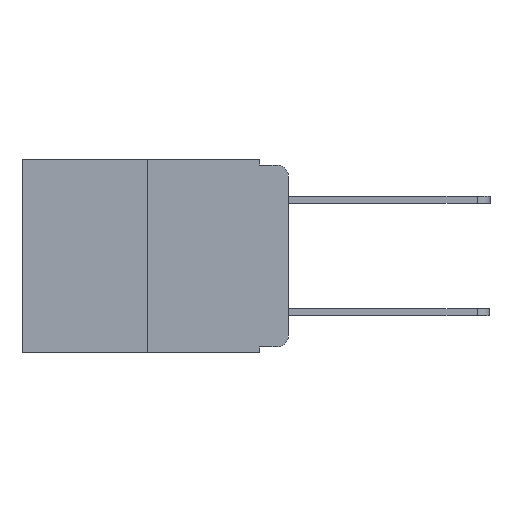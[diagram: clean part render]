
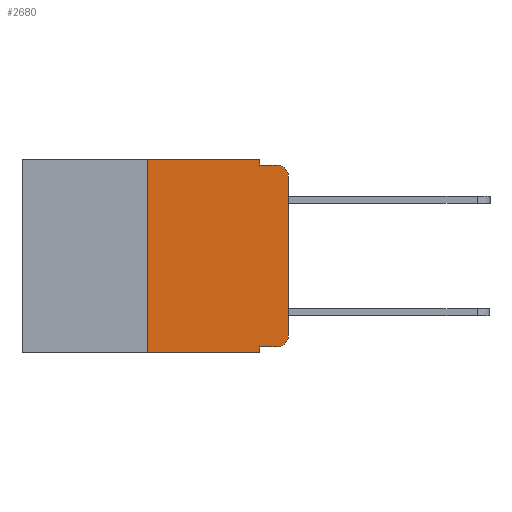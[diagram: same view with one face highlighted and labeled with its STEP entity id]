
A CAD part, left-side view. The second image highlights one B-rep face of the part: STEP entity #2680.
In plain terms, the highlighted planar face has unit normal (-1, 0, 0).
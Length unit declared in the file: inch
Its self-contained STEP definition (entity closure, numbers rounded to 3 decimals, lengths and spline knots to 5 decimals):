
#266 = DIRECTION ( 'NONE',  ( 1., 0., 0. ) ) ;
#330 = DIRECTION ( 'NONE',  ( 0., 0., -1. ) ) ;
#650 = DIRECTION ( 'NONE',  ( 0., 0., 1. ) ) ;
#925 = CARTESIAN_POINT ( 'NONE',  ( 0., 0.051, 0. ) ) ;
#1056 = CARTESIAN_POINT ( 'NONE',  ( 0., 0., -0.03 ) ) ;
#1196 = VERTEX_POINT ( 'NONE', #9554 ) ;
#1328 = CARTESIAN_POINT ( 'NONE',  ( 0., 0.02, -0.313 ) ) ;
#1429 = ORIENTED_EDGE ( 'NONE', *, *, #11269, .F. ) ;
#1903 = VECTOR ( 'NONE', #12876, 39.37008 ) ;
#2144 = CARTESIAN_POINT ( 'NONE',  ( 0., 0.051, -0.343 ) ) ;
#2455 = EDGE_LOOP ( 'NONE', ( #7905, #14167, #1429, #4999, #14502, #12250, #3129, #12959, #15816, #3548 ) ) ;
#2680 = ADVANCED_FACE ( 'NONE', ( #4405 ), #12201, .F. ) ;
#2716 = DIRECTION ( 'NONE',  ( 0., 0., -1. ) ) ;
#2804 = VECTOR ( 'NONE', #9096, 39.37008 ) ;
#2870 = CARTESIAN_POINT ( 'NONE',  ( 0., 0.25, -0.343 ) ) ;
#2989 = CARTESIAN_POINT ( 'NONE',  ( 0., 0., -0.313 ) ) ;
#3057 = CARTESIAN_POINT ( 'NONE',  ( 0., 0.25, 0. ) ) ;
#3129 = ORIENTED_EDGE ( 'NONE', *, *, #3436, .T. ) ;
#3436 = EDGE_CURVE ( 'NONE', #5664, #8452, #5036, .T. ) ;
#3548 = ORIENTED_EDGE ( 'NONE', *, *, #6524, .T. ) ;
#3634 = DIRECTION ( 'NONE',  ( 0., 0., -1. ) ) ;
#4405 = FACE_OUTER_BOUND ( 'NONE', #2455, .T. ) ;
#4482 = LINE ( 'NONE', #5975, #13395 ) ;
#4810 = CARTESIAN_POINT ( 'NONE',  ( 0., 0.051, -0.01 ) ) ;
#4999 = ORIENTED_EDGE ( 'NONE', *, *, #11222, .F. ) ;
#5036 = LINE ( 'NONE', #13894, #1903 ) ;
#5198 = VERTEX_POINT ( 'NONE', #15088 ) ;
#5568 = LINE ( 'NONE', #3057, #14623 ) ;
#5595 = EDGE_CURVE ( 'NONE', #14900, #11257, #6258, .T. ) ;
#5664 = VERTEX_POINT ( 'NONE', #2870 ) ;
#5962 = CARTESIAN_POINT ( 'NONE',  ( 0., 0.02, -0.03 ) ) ;
#5975 = CARTESIAN_POINT ( 'NONE',  ( 0., 0.051, 0. ) ) ;
#6251 = CARTESIAN_POINT ( 'NONE',  ( 0., 0.473, 0. ) ) ;
#6258 = LINE ( 'NONE', #13738, #2804 ) ;
#6524 = EDGE_CURVE ( 'NONE', #1196, #13294, #8577, .T. ) ;
#6565 = VECTOR ( 'NONE', #12065, 39.37008 ) ;
#6864 = EDGE_CURVE ( 'NONE', #5198, #1196, #7568, .T. ) ;
#7205 = DIRECTION ( 'NONE',  ( 0., 0., -1. ) ) ;
#7327 = CARTESIAN_POINT ( 'NONE',  ( 0., 0.02, -0.01 ) ) ;
#7501 = CARTESIAN_POINT ( 'NONE',  ( 0., 0.25, 0. ) ) ;
#7568 = LINE ( 'NONE', #14164, #13516 ) ;
#7828 = VERTEX_POINT ( 'NONE', #1056 ) ;
#7905 = ORIENTED_EDGE ( 'NONE', *, *, #14515, .T. ) ;
#8452 = VERTEX_POINT ( 'NONE', #2144 ) ;
#8517 = CARTESIAN_POINT ( 'NONE',  ( 0., 0.051, -0.01 ) ) ;
#8577 = CIRCLE ( 'NONE', #13328, 0.02 ) ;
#9096 = DIRECTION ( 'NONE',  ( 0., -1., 0. ) ) ;
#9297 = LINE ( 'NONE', #925, #11746 ) ;
#9554 = CARTESIAN_POINT ( 'NONE',  ( 0., 0.02, -0.333 ) ) ;
#9931 = LINE ( 'NONE', #8517, #6565 ) ;
#10249 = DIRECTION ( 'NONE',  ( -1., 0., 0. ) ) ;
#10422 = VERTEX_POINT ( 'NONE', #7327 ) ;
#10701 = EDGE_CURVE ( 'NONE', #5664, #14900, #5568, .T. ) ;
#11222 = EDGE_CURVE ( 'NONE', #11257, #14790, #4482, .T. ) ;
#11257 = VERTEX_POINT ( 'NONE', #13191 ) ;
#11269 = EDGE_CURVE ( 'NONE', #14790, #10422, #9931, .T. ) ;
#11746 = VECTOR ( 'NONE', #3634, 39.37008 ) ;
#12065 = DIRECTION ( 'NONE',  ( 0., -1., 0. ) ) ;
#12090 = AXIS2_PLACEMENT_3D ( 'NONE', #5962, #14250, #7205 ) ;
#12201 = PLANE ( 'NONE',  #12932 ) ;
#12250 = ORIENTED_EDGE ( 'NONE', *, *, #10701, .F. ) ;
#12477 = LINE ( 'NONE', #13133, #15021 ) ;
#12876 = DIRECTION ( 'NONE',  ( 0., -1., 0. ) ) ;
#12932 = AXIS2_PLACEMENT_3D ( 'NONE', #6251, #266, #330 ) ;
#12959 = ORIENTED_EDGE ( 'NONE', *, *, #15747, .F. ) ;
#13133 = CARTESIAN_POINT ( 'NONE',  ( 0., 0., 0. ) ) ;
#13191 = CARTESIAN_POINT ( 'NONE',  ( 0., 0.051, 0. ) ) ;
#13294 = VERTEX_POINT ( 'NONE', #2989 ) ;
#13328 = AXIS2_PLACEMENT_3D ( 'NONE', #1328, #10249, #2716 ) ;
#13395 = VECTOR ( 'NONE', #15309, 39.37008 ) ;
#13516 = VECTOR ( 'NONE', #15224, 39.37008 ) ;
#13738 = CARTESIAN_POINT ( 'NONE',  ( 0., 0.473, 0. ) ) ;
#13894 = CARTESIAN_POINT ( 'NONE',  ( 0., 0.473, -0.343 ) ) ;
#14164 = CARTESIAN_POINT ( 'NONE',  ( 0., 0.051, -0.333 ) ) ;
#14167 = ORIENTED_EDGE ( 'NONE', *, *, #14457, .T. ) ;
#14250 = DIRECTION ( 'NONE',  ( -1., 0., 0. ) ) ;
#14457 = EDGE_CURVE ( 'NONE', #7828, #10422, #15364, .T. ) ;
#14502 = ORIENTED_EDGE ( 'NONE', *, *, #5595, .F. ) ;
#14515 = EDGE_CURVE ( 'NONE', #13294, #7828, #12477, .T. ) ;
#14623 = VECTOR ( 'NONE', #15092, 39.37008 ) ;
#14790 = VERTEX_POINT ( 'NONE', #4810 ) ;
#14900 = VERTEX_POINT ( 'NONE', #7501 ) ;
#15021 = VECTOR ( 'NONE', #650, 39.37008 ) ;
#15088 = CARTESIAN_POINT ( 'NONE',  ( 0., 0.051, -0.333 ) ) ;
#15092 = DIRECTION ( 'NONE',  ( 0., 0., 1. ) ) ;
#15224 = DIRECTION ( 'NONE',  ( 0., -1., 0. ) ) ;
#15309 = DIRECTION ( 'NONE',  ( 0., 0., -1. ) ) ;
#15364 = CIRCLE ( 'NONE', #12090, 0.02 ) ;
#15747 = EDGE_CURVE ( 'NONE', #5198, #8452, #9297, .T. ) ;
#15816 = ORIENTED_EDGE ( 'NONE', *, *, #6864, .T. ) ;
